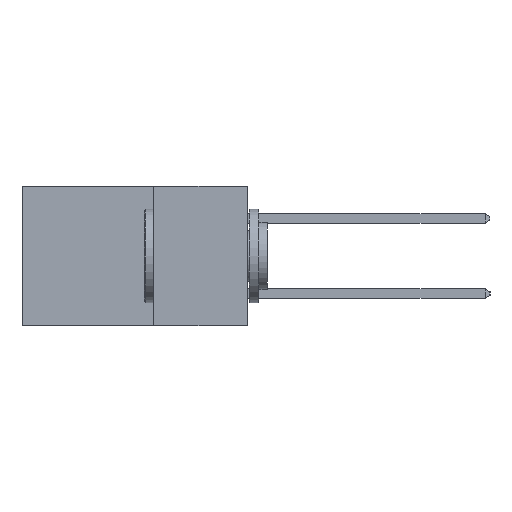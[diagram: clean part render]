
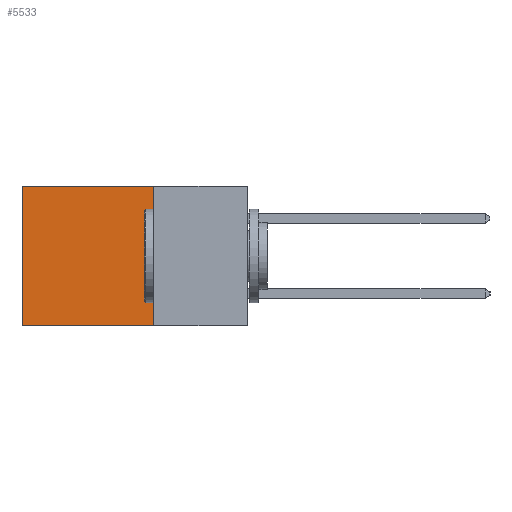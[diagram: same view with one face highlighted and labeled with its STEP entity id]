
A CAD part, left-side view. The second image highlights one B-rep face of the part: STEP entity #5533.
In plain terms, the highlighted planar face has unit normal (-1, 0, 0).
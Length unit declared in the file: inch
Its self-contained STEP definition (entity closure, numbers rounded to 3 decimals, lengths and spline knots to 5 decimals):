
#262 = ORIENTED_EDGE ( 'NONE', *, *, #773, .F. ) ;
#572 = VERTEX_POINT ( 'NONE', #9713 ) ;
#642 = VECTOR ( 'NONE', #3039, 39.37008 ) ;
#773 = EDGE_CURVE ( 'NONE', #1163, #2139, #8856, .T. ) ;
#1163 = VERTEX_POINT ( 'NONE', #10416 ) ;
#2139 = VERTEX_POINT ( 'NONE', #11217 ) ;
#2176 = LINE ( 'NONE', #2338, #4100 ) ;
#2233 = DIRECTION ( 'NONE',  ( 0., 1., 0. ) ) ;
#2338 = CARTESIAN_POINT ( 'NONE',  ( 0.2615, 0.25, 0. ) ) ;
#3039 = DIRECTION ( 'NONE',  ( 0., 0., -1. ) ) ;
#3062 = ORIENTED_EDGE ( 'NONE', *, *, #6626, .T. ) ;
#4048 = VECTOR ( 'NONE', #10620, 39.37008 ) ;
#4100 = VECTOR ( 'NONE', #2233, 39.37008 ) ;
#5003 = EDGE_LOOP ( 'NONE', ( #11992, #262, #6343, #3062 ) ) ;
#5194 = LINE ( 'NONE', #9725, #9994 ) ;
#5394 = CARTESIAN_POINT ( 'NONE',  ( 0.2615, 0.25, -0.37 ) ) ;
#5533 = ADVANCED_FACE ( 'NONE', ( #10803 ), #8141, .F. ) ;
#5617 = VERTEX_POINT ( 'NONE', #7760 ) ;
#6295 = AXIS2_PLACEMENT_3D ( 'NONE', #8102, #8061, #8059 ) ;
#6343 = ORIENTED_EDGE ( 'NONE', *, *, #11044, .F. ) ;
#6626 = EDGE_CURVE ( 'NONE', #572, #5617, #2176, .T. ) ;
#7760 = CARTESIAN_POINT ( 'NONE',  ( 0.2615, 0.6, 0. ) ) ;
#7898 = LINE ( 'NONE', #8790, #642 ) ;
#8059 = DIRECTION ( 'NONE',  ( 0., 0., -1. ) ) ;
#8061 = DIRECTION ( 'NONE',  ( 1., 0., 0. ) ) ;
#8102 = CARTESIAN_POINT ( 'NONE',  ( 0.2615, 0.25, -0.37 ) ) ;
#8141 = PLANE ( 'NONE',  #6295 ) ;
#8790 = CARTESIAN_POINT ( 'NONE',  ( 0.2615, 0.25, -0.37 ) ) ;
#8856 = LINE ( 'NONE', #5394, #4048 ) ;
#9713 = CARTESIAN_POINT ( 'NONE',  ( 0.2615, 0.25, 0. ) ) ;
#9725 = CARTESIAN_POINT ( 'NONE',  ( 0.2615, 0.6, -0.37 ) ) ;
#9767 = DIRECTION ( 'NONE',  ( 0., 0., -1. ) ) ;
#9994 = VECTOR ( 'NONE', #9767, 39.37008 ) ;
#10416 = CARTESIAN_POINT ( 'NONE',  ( 0.2615, 0.25, -0.37 ) ) ;
#10620 = DIRECTION ( 'NONE',  ( 0., 1., 0. ) ) ;
#10803 = FACE_OUTER_BOUND ( 'NONE', #5003, .T. ) ;
#11044 = EDGE_CURVE ( 'NONE', #572, #1163, #7898, .T. ) ;
#11217 = CARTESIAN_POINT ( 'NONE',  ( 0.2615, 0.6, -0.37 ) ) ;
#11738 = EDGE_CURVE ( 'NONE', #5617, #2139, #5194, .T. ) ;
#11992 = ORIENTED_EDGE ( 'NONE', *, *, #11738, .T. ) ;
